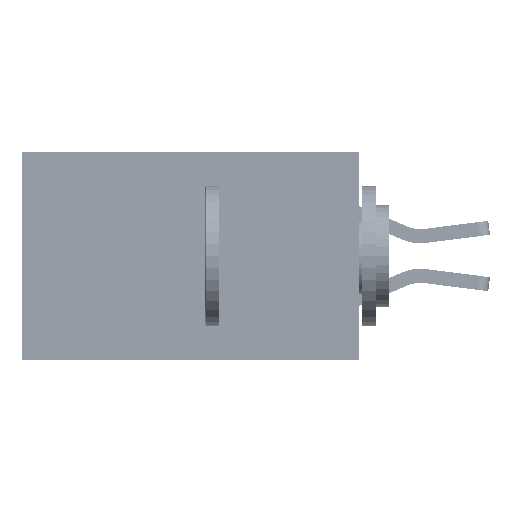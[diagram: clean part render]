
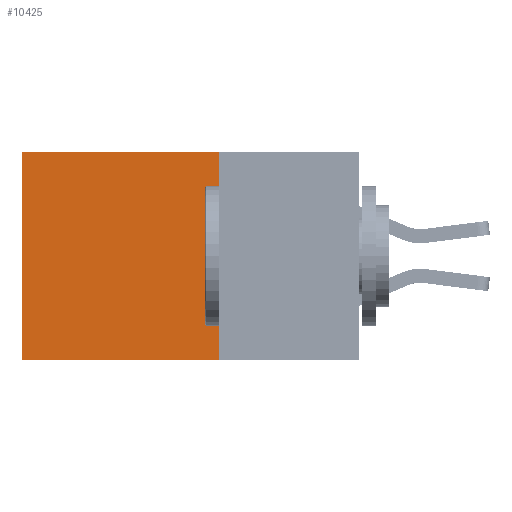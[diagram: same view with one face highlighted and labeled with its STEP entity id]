
A CAD part, left-side view. The second image highlights one B-rep face of the part: STEP entity #10425.
In plain terms, the highlighted planar face has unit normal (-1, 0, 0).
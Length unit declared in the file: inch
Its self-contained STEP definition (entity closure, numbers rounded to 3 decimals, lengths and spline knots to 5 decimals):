
#378 = VERTEX_POINT ( 'NONE', #44433 ) ;
#1062 = PLANE ( 'NONE',  #1465 ) ;
#1068 = CARTESIAN_POINT ( 'NONE',  ( 0.2875, 0.25, -0.37 ) ) ;
#1465 = AXIS2_PLACEMENT_3D ( 'NONE', #25395, #4578, #28884 ) ;
#1759 = ORIENTED_EDGE ( 'NONE', *, *, #14675, .T. ) ;
#1789 = CARTESIAN_POINT ( 'NONE',  ( 0.2875, 0.6, -0.37 ) ) ;
#3563 = EDGE_CURVE ( 'NONE', #378, #29467, #13597, .T. ) ;
#4578 = DIRECTION ( 'NONE',  ( 1., 0., 0. ) ) ;
#6480 = EDGE_CURVE ( 'NONE', #378, #32788, #20230, .T. ) ;
#8008 = VECTOR ( 'NONE', #28901, 39.37008 ) ;
#9087 = LINE ( 'NONE', #11427, #8008 ) ;
#10055 = ORIENTED_EDGE ( 'NONE', *, *, #44812, .F. ) ;
#10425 = ADVANCED_FACE ( 'NONE', ( #32328 ), #1062, .F. ) ;
#10837 = CARTESIAN_POINT ( 'NONE',  ( 0.2875, 0.25, 0. ) ) ;
#10981 = DIRECTION ( 'NONE',  ( 0., 1., 0. ) ) ;
#11427 = CARTESIAN_POINT ( 'NONE',  ( 0.2875, 0.6, 0. ) ) ;
#11574 = DIRECTION ( 'NONE',  ( 0., 0., -1. ) ) ;
#13597 = LINE ( 'NONE', #28750, #38029 ) ;
#14675 = EDGE_CURVE ( 'NONE', #32788, #26186, #9087, .T. ) ;
#19050 = CARTESIAN_POINT ( 'NONE',  ( 0.2875, 0.6, 0. ) ) ;
#19628 = LINE ( 'NONE', #1068, #35934 ) ;
#20230 = LINE ( 'NONE', #10837, #21311 ) ;
#21311 = VECTOR ( 'NONE', #10981, 39.37008 ) ;
#21375 = ORIENTED_EDGE ( 'NONE', *, *, #3563, .F. ) ;
#25395 = CARTESIAN_POINT ( 'NONE',  ( 0.2875, 0.25, 0. ) ) ;
#25871 = CARTESIAN_POINT ( 'NONE',  ( 0.2875, 0.25, -0.37 ) ) ;
#26186 = VERTEX_POINT ( 'NONE', #1789 ) ;
#28128 = ORIENTED_EDGE ( 'NONE', *, *, #6480, .T. ) ;
#28750 = CARTESIAN_POINT ( 'NONE',  ( 0.2875, 0.25, 0. ) ) ;
#28884 = DIRECTION ( 'NONE',  ( 0., 0., -1. ) ) ;
#28901 = DIRECTION ( 'NONE',  ( 0., 0., -1. ) ) ;
#29467 = VERTEX_POINT ( 'NONE', #25871 ) ;
#32328 = FACE_OUTER_BOUND ( 'NONE', #39985, .T. ) ;
#32385 = DIRECTION ( 'NONE',  ( 0., 1., 0. ) ) ;
#32788 = VERTEX_POINT ( 'NONE', #19050 ) ;
#35934 = VECTOR ( 'NONE', #32385, 39.37008 ) ;
#38029 = VECTOR ( 'NONE', #11574, 39.37008 ) ;
#39985 = EDGE_LOOP ( 'NONE', ( #1759, #10055, #21375, #28128 ) ) ;
#44433 = CARTESIAN_POINT ( 'NONE',  ( 0.2875, 0.25, 0. ) ) ;
#44812 = EDGE_CURVE ( 'NONE', #29467, #26186, #19628, .T. ) ;
